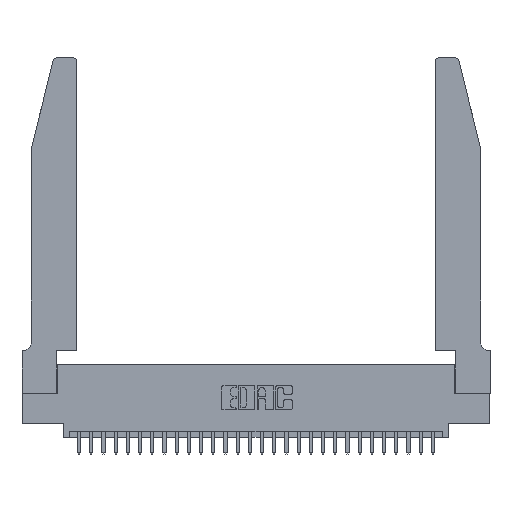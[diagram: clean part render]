
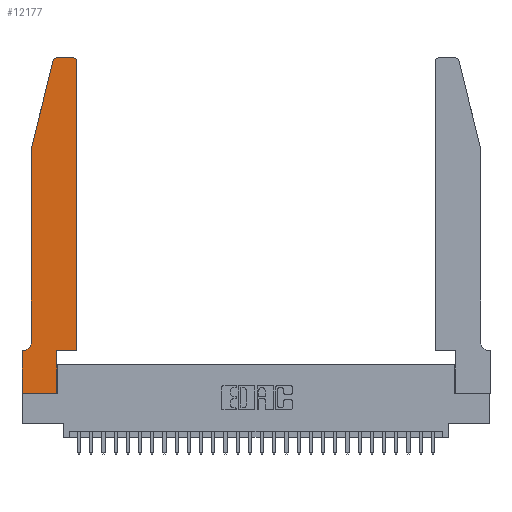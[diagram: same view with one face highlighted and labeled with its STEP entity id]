
A CAD part, top view. The second image highlights one B-rep face of the part: STEP entity #12177.
In plain terms, the highlighted planar face has unit normal (0, 0, 1).
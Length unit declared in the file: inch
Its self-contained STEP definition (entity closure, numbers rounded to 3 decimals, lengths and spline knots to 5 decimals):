
#535 = DIRECTION ( 'NONE',  ( -0.239, -0.971, 0. ) ) ;
#1002 = EDGE_CURVE ( 'NONE', #6711, #16411, #10973, .T. ) ;
#1376 = LINE ( 'NONE', #2185, #13358 ) ;
#1426 = VERTEX_POINT ( 'NONE', #18103 ) ;
#1527 = EDGE_CURVE ( 'NONE', #1426, #24216, #28736, .T. ) ;
#2185 = CARTESIAN_POINT ( 'NONE',  ( 0., 0., 0.37 ) ) ;
#2579 = CIRCLE ( 'NONE', #3567, 0.03 ) ;
#3243 = CARTESIAN_POINT ( 'NONE',  ( 0.284, 2.75, 0.37 ) ) ;
#3318 = VERTEX_POINT ( 'NONE', #20692 ) ;
#3567 = AXIS2_PLACEMENT_3D ( 'NONE', #16530, #9426, #18676 ) ;
#3602 = VECTOR ( 'NONE', #15122, 39.37008 ) ;
#3621 = VERTEX_POINT ( 'NONE', #3243 ) ;
#3889 = FACE_OUTER_BOUND ( 'NONE', #8358, .T. ) ;
#4037 = CARTESIAN_POINT ( 'NONE',  ( 0., 0.35, 0.37 ) ) ;
#4171 = ORIENTED_EDGE ( 'NONE', *, *, #11218, .T. ) ;
#4232 = DIRECTION ( 'NONE',  ( 1., 0., 0. ) ) ;
#4300 = ORIENTED_EDGE ( 'NONE', *, *, #9730, .T. ) ;
#4742 = VECTOR ( 'NONE', #23912, 39.37008 ) ;
#4863 = VERTEX_POINT ( 'NONE', #29621 ) ;
#5050 = CARTESIAN_POINT ( 'NONE',  ( 0.0755, 0.42, 0.37 ) ) ;
#5124 = VECTOR ( 'NONE', #535, 39.37008 ) ;
#5473 = CARTESIAN_POINT ( 'NONE',  ( 0.0055, 0.35, 0.37 ) ) ;
#5684 = CARTESIAN_POINT ( 'NONE',  ( 0.2865, 0.35, 0.37 ) ) ;
#6196 = ORIENTED_EDGE ( 'NONE', *, *, #14456, .T. ) ;
#6711 = VERTEX_POINT ( 'NONE', #22860 ) ;
#6810 = VERTEX_POINT ( 'NONE', #15884 ) ;
#7250 = VECTOR ( 'NONE', #27567, 39.37008 ) ;
#7499 = CARTESIAN_POINT ( 'NONE',  ( 0.4505, 0.35, 0.37 ) ) ;
#8142 = DIRECTION ( 'NONE',  ( 0., 0., -1. ) ) ;
#8358 = EDGE_LOOP ( 'NONE', ( #20386, #21334, #6196, #13342, #29763, #29628, #4300, #11435, #4171, #16013, #23803, #10334 ) ) ;
#8825 = DIRECTION ( 'NONE',  ( -1., 0., 0. ) ) ;
#9105 = VECTOR ( 'NONE', #24122, 39.37008 ) ;
#9137 = VECTOR ( 'NONE', #22244, 39.37008 ) ;
#9426 = DIRECTION ( 'NONE',  ( 0., 0., 1. ) ) ;
#9730 = EDGE_CURVE ( 'NONE', #12629, #17433, #24743, .T. ) ;
#9819 = DIRECTION ( 'NONE',  ( 0., 0., 1. ) ) ;
#9890 = CARTESIAN_POINT ( 'NONE',  ( 0.0755, 2., 0.37 ) ) ;
#10039 = CARTESIAN_POINT ( 'NONE',  ( 0.4505, 0.35, 0.37 ) ) ;
#10334 = ORIENTED_EDGE ( 'NONE', *, *, #17684, .T. ) ;
#10973 = LINE ( 'NONE', #7499, #9137 ) ;
#11218 = EDGE_CURVE ( 'NONE', #3318, #4863, #19223, .T. ) ;
#11435 = ORIENTED_EDGE ( 'NONE', *, *, #23060, .T. ) ;
#12167 = CARTESIAN_POINT ( 'NONE',  ( 0.4205, 2.75, 0.37 ) ) ;
#12177 = ADVANCED_FACE ( 'NONE', ( #3889 ), #29554, .T. ) ;
#12437 = CARTESIAN_POINT ( 'NONE',  ( 0., 0., 0.37 ) ) ;
#12629 = VERTEX_POINT ( 'NONE', #26492 ) ;
#12792 = EDGE_CURVE ( 'NONE', #4863, #6711, #29675, .T. ) ;
#13342 = ORIENTED_EDGE ( 'NONE', *, *, #1527, .T. ) ;
#13358 = VECTOR ( 'NONE', #4232, 39.37008 ) ;
#14456 = EDGE_CURVE ( 'NONE', #6810, #1426, #21106, .T. ) ;
#15122 = DIRECTION ( 'NONE',  ( 0., 1., 0. ) ) ;
#15435 = AXIS2_PLACEMENT_3D ( 'NONE', #22067, #8142, #26335 ) ;
#15757 = LINE ( 'NONE', #22729, #21950 ) ;
#15884 = CARTESIAN_POINT ( 'NONE',  ( 0.25487, 2.72718, 0.37 ) ) ;
#16013 = ORIENTED_EDGE ( 'NONE', *, *, #12792, .T. ) ;
#16367 = CARTESIAN_POINT ( 'NONE',  ( 0.0755, 0.35, 0.37 ) ) ;
#16411 = VERTEX_POINT ( 'NONE', #28484 ) ;
#16530 = CARTESIAN_POINT ( 'NONE',  ( 0.284, 2.72, 0.37 ) ) ;
#17067 = VERTEX_POINT ( 'NONE', #5473 ) ;
#17433 = VERTEX_POINT ( 'NONE', #27439 ) ;
#17661 = CIRCLE ( 'NONE', #22962, 0.03 ) ;
#17684 = EDGE_CURVE ( 'NONE', #16411, #20739, #17661, .T. ) ;
#17847 = LINE ( 'NONE', #16367, #7250 ) ;
#18103 = CARTESIAN_POINT ( 'NONE',  ( 0.0755, 2., 0.37 ) ) ;
#18676 = DIRECTION ( 'NONE',  ( 1., 0., 0. ) ) ;
#18754 = VECTOR ( 'NONE', #19087, 39.37008 ) ;
#19087 = DIRECTION ( 'NONE',  ( 1., 0., 0. ) ) ;
#19223 = LINE ( 'NONE', #5684, #3602 ) ;
#20283 = DIRECTION ( 'NONE',  ( 0., 0., 1. ) ) ;
#20386 = ORIENTED_EDGE ( 'NONE', *, *, #27625, .T. ) ;
#20692 = CARTESIAN_POINT ( 'NONE',  ( 0.2865, 0., 0.37 ) ) ;
#20739 = VERTEX_POINT ( 'NONE', #12167 ) ;
#21106 = LINE ( 'NONE', #26124, #5124 ) ;
#21334 = ORIENTED_EDGE ( 'NONE', *, *, #28687, .T. ) ;
#21950 = VECTOR ( 'NONE', #8825, 39.37008 ) ;
#22015 = EDGE_CURVE ( 'NONE', #24216, #17067, #25062, .T. ) ;
#22067 = CARTESIAN_POINT ( 'NONE',  ( 0.0055, 0.42, 0.37 ) ) ;
#22244 = DIRECTION ( 'NONE',  ( 0., 1., 0. ) ) ;
#22729 = CARTESIAN_POINT ( 'NONE',  ( 0.2605, 2.75, 0.37 ) ) ;
#22860 = CARTESIAN_POINT ( 'NONE',  ( 0.4505, 0.35, 0.37 ) ) ;
#22962 = AXIS2_PLACEMENT_3D ( 'NONE', #25985, #9819, #25874 ) ;
#23060 = EDGE_CURVE ( 'NONE', #17433, #3318, #1376, .T. ) ;
#23803 = ORIENTED_EDGE ( 'NONE', *, *, #1002, .T. ) ;
#23912 = DIRECTION ( 'NONE',  ( 0., -1., 0. ) ) ;
#24122 = DIRECTION ( 'NONE',  ( 0., -1., 0. ) ) ;
#24216 = VERTEX_POINT ( 'NONE', #5050 ) ;
#24743 = LINE ( 'NONE', #12437, #9105 ) ;
#25062 = CIRCLE ( 'NONE', #15435, 0.07 ) ;
#25874 = DIRECTION ( 'NONE',  ( 1., 0., 0. ) ) ;
#25985 = CARTESIAN_POINT ( 'NONE',  ( 0.4205, 2.72, 0.37 ) ) ;
#26124 = CARTESIAN_POINT ( 'NONE',  ( 0.0755, 2., 0.37 ) ) ;
#26335 = DIRECTION ( 'NONE',  ( -1., 0., 0. ) ) ;
#26492 = CARTESIAN_POINT ( 'NONE',  ( 0., 0.35, 0.37 ) ) ;
#27439 = CARTESIAN_POINT ( 'NONE',  ( 0., 0., 0.37 ) ) ;
#27567 = DIRECTION ( 'NONE',  ( -1., 0., 0. ) ) ;
#27625 = EDGE_CURVE ( 'NONE', #20739, #3621, #15757, .T. ) ;
#27728 = AXIS2_PLACEMENT_3D ( 'NONE', #4037, #20283, #29641 ) ;
#28484 = CARTESIAN_POINT ( 'NONE',  ( 0.4505, 2.72, 0.37 ) ) ;
#28687 = EDGE_CURVE ( 'NONE', #3621, #6810, #2579, .T. ) ;
#28736 = LINE ( 'NONE', #9890, #4742 ) ;
#29554 = PLANE ( 'NONE',  #27728 ) ;
#29621 = CARTESIAN_POINT ( 'NONE',  ( 0.2865, 0.35, 0.37 ) ) ;
#29628 = ORIENTED_EDGE ( 'NONE', *, *, #29894, .T. ) ;
#29641 = DIRECTION ( 'NONE',  ( 1., 0., 0. ) ) ;
#29675 = LINE ( 'NONE', #10039, #18754 ) ;
#29763 = ORIENTED_EDGE ( 'NONE', *, *, #22015, .T. ) ;
#29894 = EDGE_CURVE ( 'NONE', #17067, #12629, #17847, .T. ) ;
